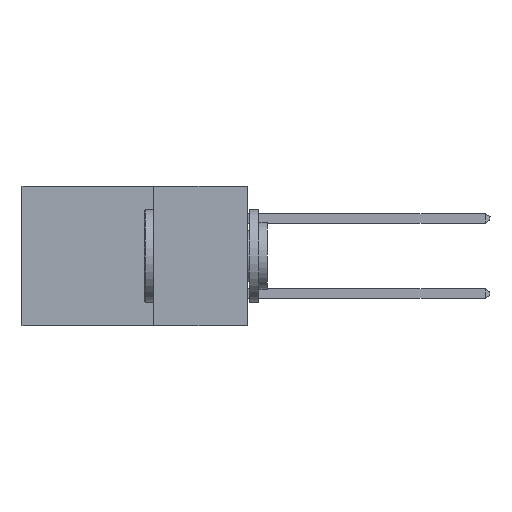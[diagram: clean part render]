
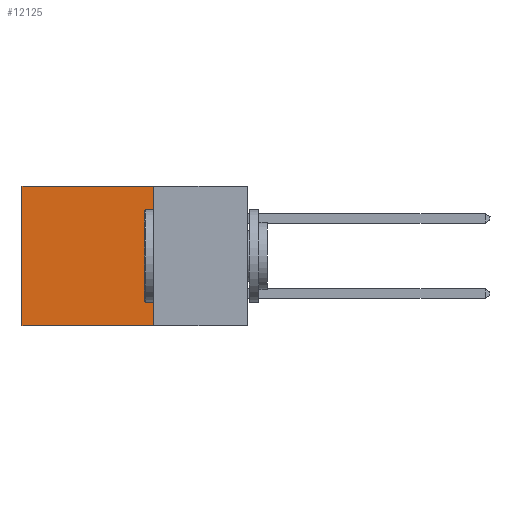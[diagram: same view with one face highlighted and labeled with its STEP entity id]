
A CAD part, left-side view. The second image highlights one B-rep face of the part: STEP entity #12125.
In plain terms, the highlighted planar face has unit normal (-1, 0, 0).
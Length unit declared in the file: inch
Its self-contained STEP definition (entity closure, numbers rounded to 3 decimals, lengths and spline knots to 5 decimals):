
#35 = ORIENTED_EDGE ( 'NONE', *, *, #10495, .F. ) ;
#1189 = EDGE_CURVE ( 'NONE', #20454, #2314, #27477, .T. ) ;
#1499 = CARTESIAN_POINT ( 'NONE',  ( 0.298, 0.25, 0. ) ) ;
#2314 = VERTEX_POINT ( 'NONE', #4941 ) ;
#2511 = VERTEX_POINT ( 'NONE', #10045 ) ;
#3268 = LINE ( 'NONE', #23389, #9832 ) ;
#3971 = ORIENTED_EDGE ( 'NONE', *, *, #22334, .T. ) ;
#4941 = CARTESIAN_POINT ( 'NONE',  ( 0.298, 0.6, 0. ) ) ;
#7719 = CARTESIAN_POINT ( 'NONE',  ( 0.298, 0.6, 0. ) ) ;
#7981 = LINE ( 'NONE', #7719, #20106 ) ;
#8115 = FACE_OUTER_BOUND ( 'NONE', #13257, .T. ) ;
#9027 = EDGE_CURVE ( 'NONE', #20454, #29047, #3268, .T. ) ;
#9832 = VECTOR ( 'NONE', #24057, 39.37008 ) ;
#10045 = CARTESIAN_POINT ( 'NONE',  ( 0.298, 0.6, -0.37 ) ) ;
#10146 = DIRECTION ( 'NONE',  ( 0., 0., -1. ) ) ;
#10495 = EDGE_CURVE ( 'NONE', #29047, #2511, #16567, .T. ) ;
#12125 = ADVANCED_FACE ( 'NONE', ( #8115 ), #13855, .F. ) ;
#13257 = EDGE_LOOP ( 'NONE', ( #3971, #35, #16669, #17951 ) ) ;
#13855 = PLANE ( 'NONE',  #24590 ) ;
#16316 = DIRECTION ( 'NONE',  ( 0., 0., -1. ) ) ;
#16567 = LINE ( 'NONE', #25766, #22947 ) ;
#16669 = ORIENTED_EDGE ( 'NONE', *, *, #9027, .F. ) ;
#17951 = ORIENTED_EDGE ( 'NONE', *, *, #1189, .T. ) ;
#20106 = VECTOR ( 'NONE', #10146, 39.37008 ) ;
#20454 = VERTEX_POINT ( 'NONE', #30145 ) ;
#21192 = VECTOR ( 'NONE', #29134, 39.37008 ) ;
#21691 = CARTESIAN_POINT ( 'NONE',  ( 0.298, 0.25, 0. ) ) ;
#22334 = EDGE_CURVE ( 'NONE', #2314, #2511, #7981, .T. ) ;
#22947 = VECTOR ( 'NONE', #25628, 39.37008 ) ;
#23389 = CARTESIAN_POINT ( 'NONE',  ( 0.298, 0.25, 0. ) ) ;
#24057 = DIRECTION ( 'NONE',  ( 0., 0., -1. ) ) ;
#24590 = AXIS2_PLACEMENT_3D ( 'NONE', #1499, #30528, #16316 ) ;
#25628 = DIRECTION ( 'NONE',  ( 0., 1., 0. ) ) ;
#25766 = CARTESIAN_POINT ( 'NONE',  ( 0.298, 0.25, -0.37 ) ) ;
#27465 = CARTESIAN_POINT ( 'NONE',  ( 0.298, 0.25, -0.37 ) ) ;
#27477 = LINE ( 'NONE', #21691, #21192 ) ;
#29047 = VERTEX_POINT ( 'NONE', #27465 ) ;
#29134 = DIRECTION ( 'NONE',  ( 0., 1., 0. ) ) ;
#30145 = CARTESIAN_POINT ( 'NONE',  ( 0.298, 0.25, 0. ) ) ;
#30528 = DIRECTION ( 'NONE',  ( 1., 0., 0. ) ) ;
